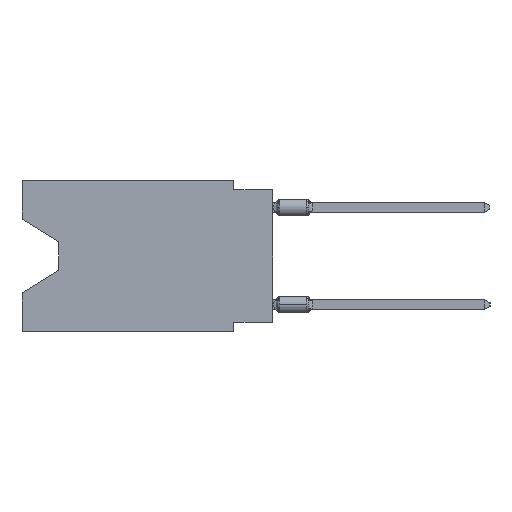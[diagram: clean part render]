
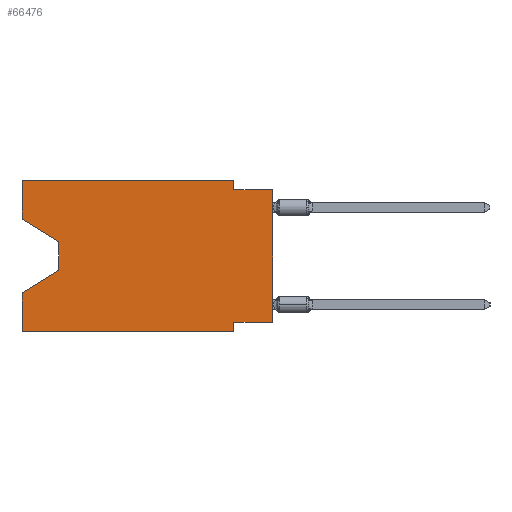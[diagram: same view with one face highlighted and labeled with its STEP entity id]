
A CAD part, left-side view. The second image highlights one B-rep face of the part: STEP entity #66476.
In plain terms, the highlighted planar face has unit normal (-1, 0, 0).
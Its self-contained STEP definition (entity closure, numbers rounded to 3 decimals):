
#116 = LINE ( 'NONE', #58963, #5164 ) ;
#173 = ORIENTED_EDGE ( 'NONE', *, *, #40421, .F. ) ;
#297 = CARTESIAN_POINT ( 'NONE',  ( 0., 0., -0.635 ) ) ;
#1958 = VERTEX_POINT ( 'NONE', #11959 ) ;
#2411 = DIRECTION ( 'NONE',  ( 0., 0., -1. ) ) ;
#2680 = VERTEX_POINT ( 'NONE', #45207 ) ;
#4295 = ORIENTED_EDGE ( 'NONE', *, *, #56663, .F. ) ;
#5164 = VECTOR ( 'NONE', #22348, 1000. ) ;
#5909 = CARTESIAN_POINT ( 'NONE',  ( 0., 2.54, -9.906 ) ) ;
#6277 = ORIENTED_EDGE ( 'NONE', *, *, #41430, .F. ) ;
#6416 = EDGE_CURVE ( 'NONE', #52086, #43097, #59722, .T. ) ;
#7208 = ORIENTED_EDGE ( 'NONE', *, *, #48442, .T. ) ;
#7297 = VECTOR ( 'NONE', #55451, 1000. ) ;
#7492 = VECTOR ( 'NONE', #2411, 1000. ) ;
#7646 = VECTOR ( 'NONE', #39405, 1000. ) ;
#7686 = EDGE_CURVE ( 'NONE', #1958, #59828, #44679, .T. ) ;
#7844 = CARTESIAN_POINT ( 'NONE',  ( 0., 16.383, -2.546 ) ) ;
#7845 = CARTESIAN_POINT ( 'NONE',  ( 0., 16.383, 0. ) ) ;
#10154 = AXIS2_PLACEMENT_3D ( 'NONE', #7845, #17788, #28749 ) ;
#11959 = CARTESIAN_POINT ( 'NONE',  ( 0., 13.97, -4.013 ) ) ;
#12680 = LINE ( 'NONE', #43483, #7492 ) ;
#13706 = LINE ( 'NONE', #34576, #7297 ) ;
#14436 = EDGE_CURVE ( 'NONE', #52086, #2680, #65408, .T. ) ;
#15391 = VERTEX_POINT ( 'NONE', #50848 ) ;
#15512 = LINE ( 'NONE', #5909, #18051 ) ;
#17788 = DIRECTION ( 'NONE',  ( 1., 0., 0. ) ) ;
#18051 = VECTOR ( 'NONE', #62740, 1000. ) ;
#19621 = ORIENTED_EDGE ( 'NONE', *, *, #7686, .T. ) ;
#19637 = CARTESIAN_POINT ( 'NONE',  ( 0., 16.383, -9.906 ) ) ;
#21011 = ORIENTED_EDGE ( 'NONE', *, *, #33360, .F. ) ;
#22348 = DIRECTION ( 'NONE',  ( 0., 0.855, -0.519 ) ) ;
#22459 = ORIENTED_EDGE ( 'NONE', *, *, #57039, .T. ) ;
#22502 = CARTESIAN_POINT ( 'NONE',  ( 0., 16.383, -9.906 ) ) ;
#24472 = CARTESIAN_POINT ( 'NONE',  ( 0., 0., -9.271 ) ) ;
#26363 = ORIENTED_EDGE ( 'NONE', *, *, #14436, .T. ) ;
#26662 = DIRECTION ( 'NONE',  ( 0., -1., 0. ) ) ;
#27780 = ORIENTED_EDGE ( 'NONE', *, *, #66866, .T. ) ;
#28749 = DIRECTION ( 'NONE',  ( 0., 0., -1. ) ) ;
#28907 = VERTEX_POINT ( 'NONE', #40248 ) ;
#30990 = VECTOR ( 'NONE', #48858, 1000. ) ;
#31027 = LINE ( 'NONE', #51895, #47864 ) ;
#32200 = VERTEX_POINT ( 'NONE', #33722 ) ;
#33360 = EDGE_CURVE ( 'NONE', #65334, #2680, #52330, .T. ) ;
#33722 = CARTESIAN_POINT ( 'NONE',  ( 0., 16.383, 0. ) ) ;
#33736 = DIRECTION ( 'NONE',  ( 0., 0., -1. ) ) ;
#33954 = ORIENTED_EDGE ( 'NONE', *, *, #37204, .F. ) ;
#34576 = CARTESIAN_POINT ( 'NONE',  ( 0., 16.383, 0. ) ) ;
#35615 = VECTOR ( 'NONE', #26662, 1000. ) ;
#35634 = CARTESIAN_POINT ( 'NONE',  ( 0., 0., -9.271 ) ) ;
#37204 = EDGE_CURVE ( 'NONE', #32200, #15391, #13706, .T. ) ;
#37494 = CARTESIAN_POINT ( 'NONE',  ( 0., 16.383, 0. ) ) ;
#38372 = CARTESIAN_POINT ( 'NONE',  ( 0., 0., 0. ) ) ;
#39405 = DIRECTION ( 'NONE',  ( 0., 0., 1. ) ) ;
#40248 = CARTESIAN_POINT ( 'NONE',  ( 0., 16.383, -7.36 ) ) ;
#40421 = EDGE_CURVE ( 'NONE', #60862, #32200, #31027, .T. ) ;
#40717 = CARTESIAN_POINT ( 'NONE',  ( 0., 16.383, -2.546 ) ) ;
#41430 = EDGE_CURVE ( 'NONE', #15391, #65334, #12680, .T. ) ;
#42051 = CARTESIAN_POINT ( 'NONE',  ( 0., 13.97, -5.893 ) ) ;
#42751 = EDGE_LOOP ( 'NONE', ( #7208, #19621, #22459, #4295, #27780, #56309, #47150, #26363, #21011, #6277, #33954, #173 ) ) ;
#43097 = VERTEX_POINT ( 'NONE', #47839 ) ;
#43483 = CARTESIAN_POINT ( 'NONE',  ( 0., 2.54, 0. ) ) ;
#43603 = VECTOR ( 'NONE', #33736, 1000. ) ;
#44679 = LINE ( 'NONE', #66215, #43603 ) ;
#45050 = VERTEX_POINT ( 'NONE', #55916 ) ;
#45207 = CARTESIAN_POINT ( 'NONE',  ( 0., 0., -0.635 ) ) ;
#45342 = DIRECTION ( 'NONE',  ( 0., 1., 0. ) ) ;
#45863 = VECTOR ( 'NONE', #45342, 1000. ) ;
#47150 = ORIENTED_EDGE ( 'NONE', *, *, #6416, .F. ) ;
#47839 = CARTESIAN_POINT ( 'NONE',  ( 0., 2.54, -9.271 ) ) ;
#47864 = VECTOR ( 'NONE', #56694, 1000. ) ;
#48442 = EDGE_CURVE ( 'NONE', #60862, #1958, #59869, .T. ) ;
#48858 = DIRECTION ( 'NONE',  ( 0., -1., 0. ) ) ;
#49611 = DIRECTION ( 'NONE',  ( 0., -0.855, -0.519 ) ) ;
#50848 = CARTESIAN_POINT ( 'NONE',  ( 0., 2.54, 0. ) ) ;
#51800 = EDGE_CURVE ( 'NONE', #43097, #45050, #15512, .T. ) ;
#51895 = CARTESIAN_POINT ( 'NONE',  ( 0., 16.383, 0. ) ) ;
#52086 = VERTEX_POINT ( 'NONE', #35634 ) ;
#52330 = LINE ( 'NONE', #297, #35615 ) ;
#55451 = DIRECTION ( 'NONE',  ( 0., -1., 0. ) ) ;
#55459 = VECTOR ( 'NONE', #64176, 1000. ) ;
#55834 = VERTEX_POINT ( 'NONE', #19637 ) ;
#55916 = CARTESIAN_POINT ( 'NONE',  ( 0., 2.54, -9.906 ) ) ;
#56309 = ORIENTED_EDGE ( 'NONE', *, *, #51800, .F. ) ;
#56663 = EDGE_CURVE ( 'NONE', #55834, #28907, #61144, .T. ) ;
#56694 = DIRECTION ( 'NONE',  ( 0., 0., 1. ) ) ;
#57039 = EDGE_CURVE ( 'NONE', #59828, #28907, #116, .T. ) ;
#58963 = CARTESIAN_POINT ( 'NONE',  ( 0., 13.97, -5.893 ) ) ;
#59722 = LINE ( 'NONE', #24472, #45863 ) ;
#59828 = VERTEX_POINT ( 'NONE', #42051 ) ;
#59869 = LINE ( 'NONE', #7844, #67152 ) ;
#60210 = FACE_OUTER_BOUND ( 'NONE', #42751, .T. ) ;
#60862 = VERTEX_POINT ( 'NONE', #40717 ) ;
#61144 = LINE ( 'NONE', #37494, #55459 ) ;
#62740 = DIRECTION ( 'NONE',  ( 0., 0., -1. ) ) ;
#64176 = DIRECTION ( 'NONE',  ( 0., 0., 1. ) ) ;
#64670 = PLANE ( 'NONE',  #10154 ) ;
#64832 = CARTESIAN_POINT ( 'NONE',  ( 0., 2.54, -0.635 ) ) ;
#65334 = VERTEX_POINT ( 'NONE', #64832 ) ;
#65408 = LINE ( 'NONE', #38372, #7646 ) ;
#65605 = LINE ( 'NONE', #22502, #30990 ) ;
#66215 = CARTESIAN_POINT ( 'NONE',  ( 0., 13.97, -4.013 ) ) ;
#66476 = ADVANCED_FACE ( 'NONE', ( #60210 ), #64670, .F. ) ;
#66866 = EDGE_CURVE ( 'NONE', #55834, #45050, #65605, .T. ) ;
#67152 = VECTOR ( 'NONE', #49611, 1000. ) ;
